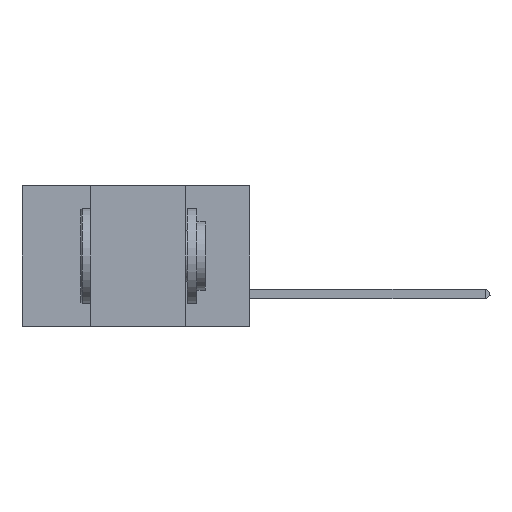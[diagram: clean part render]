
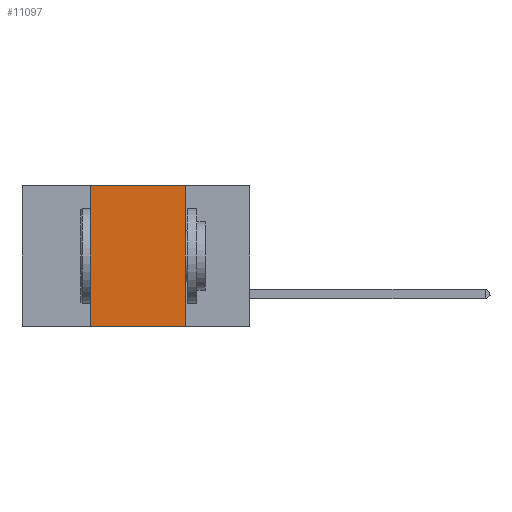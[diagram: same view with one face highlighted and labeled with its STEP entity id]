
A CAD part, left-side view. The second image highlights one B-rep face of the part: STEP entity #11097.
In plain terms, the highlighted planar face has unit normal (-1, 0, 0).
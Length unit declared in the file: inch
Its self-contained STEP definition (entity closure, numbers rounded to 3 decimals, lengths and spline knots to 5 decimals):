
#765 = CARTESIAN_POINT ( 'NONE',  ( 0., 0.42, 0. ) ) ;
#830 = VERTEX_POINT ( 'NONE', #18834 ) ;
#1846 = CARTESIAN_POINT ( 'NONE',  ( 0., 0.6, 0. ) ) ;
#1948 = LINE ( 'NONE', #8086, #17977 ) ;
#2628 = CARTESIAN_POINT ( 'NONE',  ( 0., 0.6, 0. ) ) ;
#2819 = DIRECTION ( 'NONE',  ( 0., -1., 0. ) ) ;
#4220 = VECTOR ( 'NONE', #13166, 39.37008 ) ;
#4783 = ORIENTED_EDGE ( 'NONE', *, *, #16110, .F. ) ;
#5673 = CARTESIAN_POINT ( 'NONE',  ( 0., 0.42, -0.37 ) ) ;
#5680 = CARTESIAN_POINT ( 'NONE',  ( 0., 0.17, 0. ) ) ;
#6141 = FACE_OUTER_BOUND ( 'NONE', #11907, .T. ) ;
#6500 = ORIENTED_EDGE ( 'NONE', *, *, #13400, .F. ) ;
#7688 = LINE ( 'NONE', #20003, #16658 ) ;
#7944 = DIRECTION ( 'NONE',  ( 1., 0., 0. ) ) ;
#8086 = CARTESIAN_POINT ( 'NONE',  ( 0., 0.17, 0. ) ) ;
#8218 = DIRECTION ( 'NONE',  ( 0., 0., -1. ) ) ;
#9472 = DIRECTION ( 'NONE',  ( 0., 0., -1. ) ) ;
#10475 = EDGE_CURVE ( 'NONE', #11548, #19538, #18070, .T. ) ;
#10925 = DIRECTION ( 'NONE',  ( 0., -1., 0. ) ) ;
#11069 = PLANE ( 'NONE',  #15322 ) ;
#11097 = ADVANCED_FACE ( 'NONE', ( #6141 ), #11069, .F. ) ;
#11215 = ORIENTED_EDGE ( 'NONE', *, *, #19834, .T. ) ;
#11548 = VERTEX_POINT ( 'NONE', #5673 ) ;
#11756 = LINE ( 'NONE', #2628, #18063 ) ;
#11907 = EDGE_LOOP ( 'NONE', ( #6500, #4783, #14253, #11215 ) ) ;
#13166 = DIRECTION ( 'NONE',  ( 0., 0., 1. ) ) ;
#13400 = EDGE_CURVE ( 'NONE', #18368, #830, #1948, .T. ) ;
#14253 = ORIENTED_EDGE ( 'NONE', *, *, #10475, .F. ) ;
#15322 = AXIS2_PLACEMENT_3D ( 'NONE', #1846, #7944, #9472 ) ;
#16110 = EDGE_CURVE ( 'NONE', #19538, #18368, #11756, .T. ) ;
#16658 = VECTOR ( 'NONE', #10925, 39.37008 ) ;
#16830 = CARTESIAN_POINT ( 'NONE',  ( 0., 0.42, 0. ) ) ;
#17977 = VECTOR ( 'NONE', #8218, 39.37008 ) ;
#18063 = VECTOR ( 'NONE', #2819, 39.37008 ) ;
#18070 = LINE ( 'NONE', #765, #4220 ) ;
#18368 = VERTEX_POINT ( 'NONE', #5680 ) ;
#18834 = CARTESIAN_POINT ( 'NONE',  ( 0., 0.17, -0.37 ) ) ;
#19538 = VERTEX_POINT ( 'NONE', #16830 ) ;
#19834 = EDGE_CURVE ( 'NONE', #11548, #830, #7688, .T. ) ;
#20003 = CARTESIAN_POINT ( 'NONE',  ( 0., 0.6, -0.37 ) ) ;
